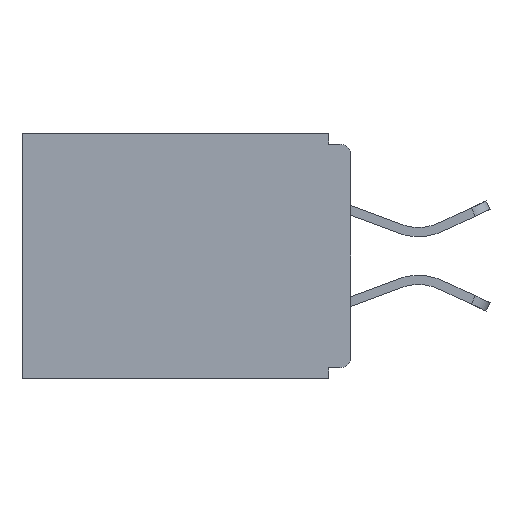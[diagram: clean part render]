
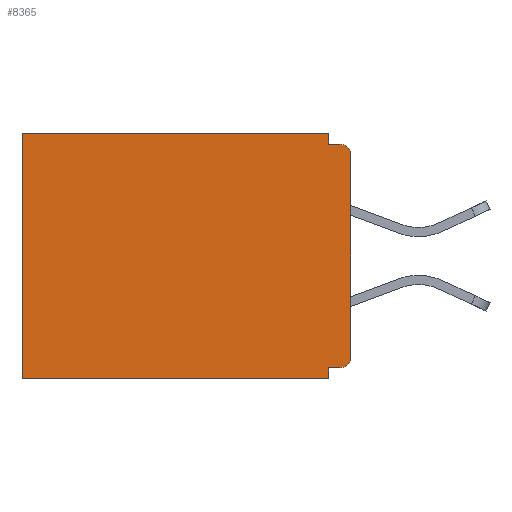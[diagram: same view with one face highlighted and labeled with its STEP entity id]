
A CAD part, left-side view. The second image highlights one B-rep face of the part: STEP entity #8365.
In plain terms, the highlighted planar face has unit normal (-1, 0, 0).
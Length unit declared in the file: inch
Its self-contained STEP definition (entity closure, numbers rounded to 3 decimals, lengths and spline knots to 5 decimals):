
#6 = ORIENTED_EDGE ( 'NONE', *, *, #23355, .T. ) ;
#43 = ORIENTED_EDGE ( 'NONE', *, *, #16621, .F. ) ;
#213 = DIRECTION ( 'NONE',  ( 0., 0., -1. ) ) ;
#317 = DIRECTION ( 'NONE',  ( 0., 1., 0. ) ) ;
#1537 = CARTESIAN_POINT ( 'NONE',  ( 0.298, 0., -0.03 ) ) ;
#2536 = VERTEX_POINT ( 'NONE', #21208 ) ;
#2939 = ORIENTED_EDGE ( 'NONE', *, *, #13980, .F. ) ;
#3111 = VECTOR ( 'NONE', #19022, 39.37008 ) ;
#3164 = CARTESIAN_POINT ( 'NONE',  ( 0.298, 0., -0.328 ) ) ;
#3201 = CARTESIAN_POINT ( 'NONE',  ( 0.298, 0., 0. ) ) ;
#3352 = CARTESIAN_POINT ( 'NONE',  ( 0.298, 0.031, 0. ) ) ;
#3602 = VECTOR ( 'NONE', #20649, 39.37008 ) ;
#3607 = CARTESIAN_POINT ( 'NONE',  ( 0.298, 0.015, -0.328 ) ) ;
#3669 = VERTEX_POINT ( 'NONE', #21573 ) ;
#4017 = VECTOR ( 'NONE', #317, 39.37008 ) ;
#4042 = EDGE_CURVE ( 'NONE', #5870, #3669, #6302, .T. ) ;
#4706 = LINE ( 'NONE', #9533, #3602 ) ;
#4843 = EDGE_CURVE ( 'NONE', #18484, #13876, #16292, .T. ) ;
#4872 = LINE ( 'NONE', #13456, #4017 ) ;
#5022 = DIRECTION ( 'NONE',  ( 0., 1., 0. ) ) ;
#5067 = DIRECTION ( 'NONE',  ( 1., 0., 0. ) ) ;
#5287 = ORIENTED_EDGE ( 'NONE', *, *, #11186, .F. ) ;
#5454 = LINE ( 'NONE', #7679, #18038 ) ;
#5642 = DIRECTION ( 'NONE',  ( 0., 1., 0. ) ) ;
#5870 = VERTEX_POINT ( 'NONE', #8566 ) ;
#5875 = DIRECTION ( 'NONE',  ( -1., 0., 0. ) ) ;
#5964 = LINE ( 'NONE', #9646, #23030 ) ;
#6024 = CARTESIAN_POINT ( 'NONE',  ( 0.298, 0.015, -0.313 ) ) ;
#6302 = LINE ( 'NONE', #22899, #3111 ) ;
#6405 = ORIENTED_EDGE ( 'NONE', *, *, #6699, .F. ) ;
#6433 = CIRCLE ( 'NONE', #14954, 0.015 ) ;
#6542 = DIRECTION ( 'NONE',  ( -1., 0., 0. ) ) ;
#6609 = VERTEX_POINT ( 'NONE', #21657 ) ;
#6699 = EDGE_CURVE ( 'NONE', #6790, #2536, #23299, .T. ) ;
#6790 = VERTEX_POINT ( 'NONE', #3352 ) ;
#7310 = CARTESIAN_POINT ( 'NONE',  ( 0.298, 0.46, 0. ) ) ;
#7514 = AXIS2_PLACEMENT_3D ( 'NONE', #3201, #5067, #8746 ) ;
#7595 = EDGE_CURVE ( 'NONE', #2536, #6609, #4706, .T. ) ;
#7679 = CARTESIAN_POINT ( 'NONE',  ( 0.298, 0., -0.343 ) ) ;
#8365 = ADVANCED_FACE ( 'NONE', ( #17322 ), #19864, .F. ) ;
#8566 = CARTESIAN_POINT ( 'NONE',  ( 0.298, 0.031, -0.328 ) ) ;
#8746 = DIRECTION ( 'NONE',  ( 0., 0., -1. ) ) ;
#9235 = ORIENTED_EDGE ( 'NONE', *, *, #22527, .T. ) ;
#9354 = CIRCLE ( 'NONE', #11492, 0.015 ) ;
#9533 = CARTESIAN_POINT ( 'NONE',  ( 0.298, 0., -0.015 ) ) ;
#9646 = CARTESIAN_POINT ( 'NONE',  ( 0.298, 0., 0. ) ) ;
#10881 = CARTESIAN_POINT ( 'NONE',  ( 0.298, 0.031, -0.343 ) ) ;
#11186 = EDGE_CURVE ( 'NONE', #3669, #13876, #5454, .T. ) ;
#11226 = VERTEX_POINT ( 'NONE', #3607 ) ;
#11492 = AXIS2_PLACEMENT_3D ( 'NONE', #6024, #5875, #19178 ) ;
#13203 = VECTOR ( 'NONE', #5022, 39.37008 ) ;
#13456 = CARTESIAN_POINT ( 'NONE',  ( 0.298, 0., 0. ) ) ;
#13553 = CARTESIAN_POINT ( 'NONE',  ( 0.298, 0.46, -0.343 ) ) ;
#13876 = VERTEX_POINT ( 'NONE', #13553 ) ;
#13980 = EDGE_CURVE ( 'NONE', #16208, #17982, #5964, .T. ) ;
#14954 = AXIS2_PLACEMENT_3D ( 'NONE', #19547, #6542, #17788 ) ;
#16208 = VERTEX_POINT ( 'NONE', #1537 ) ;
#16292 = LINE ( 'NONE', #7310, #21891 ) ;
#16296 = ORIENTED_EDGE ( 'NONE', *, *, #7595, .F. ) ;
#16621 = EDGE_CURVE ( 'NONE', #11226, #5870, #23466, .T. ) ;
#17322 = FACE_OUTER_BOUND ( 'NONE', #18096, .T. ) ;
#17788 = DIRECTION ( 'NONE',  ( 0., 0., -1. ) ) ;
#17982 = VERTEX_POINT ( 'NONE', #22461 ) ;
#18038 = VECTOR ( 'NONE', #5642, 39.37008 ) ;
#18096 = EDGE_LOOP ( 'NONE', ( #22412, #16296, #6405, #6, #21204, #5287, #23540, #43, #9235, #2939 ) ) ;
#18484 = VERTEX_POINT ( 'NONE', #20124 ) ;
#19022 = DIRECTION ( 'NONE',  ( 0., 0., -1. ) ) ;
#19178 = DIRECTION ( 'NONE',  ( 0., 0., -1. ) ) ;
#19547 = CARTESIAN_POINT ( 'NONE',  ( 0.298, 0.015, -0.03 ) ) ;
#19864 = PLANE ( 'NONE',  #7514 ) ;
#20124 = CARTESIAN_POINT ( 'NONE',  ( 0.298, 0.46, 0. ) ) ;
#20464 = DIRECTION ( 'NONE',  ( 0., 0., -1. ) ) ;
#20649 = DIRECTION ( 'NONE',  ( 0., -1., 0. ) ) ;
#21204 = ORIENTED_EDGE ( 'NONE', *, *, #4843, .T. ) ;
#21208 = CARTESIAN_POINT ( 'NONE',  ( 0.298, 0.031, -0.015 ) ) ;
#21573 = CARTESIAN_POINT ( 'NONE',  ( 0.298, 0.031, -0.343 ) ) ;
#21657 = CARTESIAN_POINT ( 'NONE',  ( 0.298, 0.015, -0.015 ) ) ;
#21769 = EDGE_CURVE ( 'NONE', #16208, #6609, #6433, .T. ) ;
#21891 = VECTOR ( 'NONE', #20464, 39.37008 ) ;
#22412 = ORIENTED_EDGE ( 'NONE', *, *, #21769, .T. ) ;
#22461 = CARTESIAN_POINT ( 'NONE',  ( 0.298, 0., -0.313 ) ) ;
#22527 = EDGE_CURVE ( 'NONE', #11226, #17982, #9354, .T. ) ;
#22754 = VECTOR ( 'NONE', #23971, 39.37008 ) ;
#22899 = CARTESIAN_POINT ( 'NONE',  ( 0.298, 0.031, -0.343 ) ) ;
#23030 = VECTOR ( 'NONE', #213, 39.37008 ) ;
#23299 = LINE ( 'NONE', #10881, #22754 ) ;
#23355 = EDGE_CURVE ( 'NONE', #6790, #18484, #4872, .T. ) ;
#23466 = LINE ( 'NONE', #3164, #13203 ) ;
#23540 = ORIENTED_EDGE ( 'NONE', *, *, #4042, .F. ) ;
#23971 = DIRECTION ( 'NONE',  ( 0., 0., -1. ) ) ;
